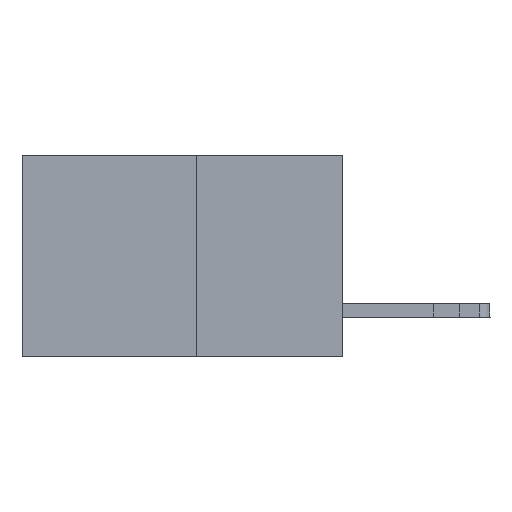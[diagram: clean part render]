
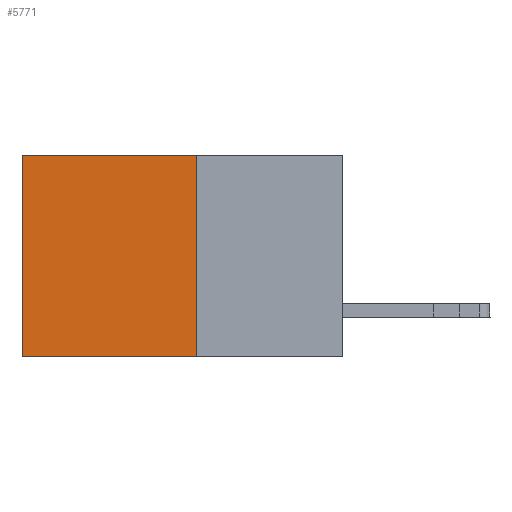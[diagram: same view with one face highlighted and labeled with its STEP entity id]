
A CAD part, left-side view. The second image highlights one B-rep face of the part: STEP entity #5771.
In plain terms, the highlighted planar face has unit normal (-1, 0, 0).
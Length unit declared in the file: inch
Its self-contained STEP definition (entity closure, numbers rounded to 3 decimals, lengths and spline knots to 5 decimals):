
#419 = FACE_OUTER_BOUND ( 'NONE', #8455, .T. ) ;
#1815 = LINE ( 'NONE', #14845, #19613 ) ;
#2249 = VERTEX_POINT ( 'NONE', #11006 ) ;
#2695 = CARTESIAN_POINT ( 'NONE',  ( 0.277, 0.27, -0.37 ) ) ;
#3165 = EDGE_CURVE ( 'NONE', #24280, #2249, #1815, .T. ) ;
#3408 = CARTESIAN_POINT ( 'NONE',  ( 0.277, 0.59, -0.37 ) ) ;
#4039 = EDGE_CURVE ( 'NONE', #24280, #22202, #10521, .T. ) ;
#5771 = ADVANCED_FACE ( 'NONE', ( #419 ), #15603, .F. ) ;
#6904 = LINE ( 'NONE', #11055, #23660 ) ;
#7126 = CARTESIAN_POINT ( 'NONE',  ( 0.277, 0.27, -0.37 ) ) ;
#8455 = EDGE_LOOP ( 'NONE', ( #21153, #15547, #9167, #14128 ) ) ;
#9142 = DIRECTION ( 'NONE',  ( 0., 1., 0. ) ) ;
#9167 = ORIENTED_EDGE ( 'NONE', *, *, #4039, .F. ) ;
#10252 = EDGE_CURVE ( 'NONE', #2249, #18448, #6904, .T. ) ;
#10521 = LINE ( 'NONE', #2695, #21173 ) ;
#11006 = CARTESIAN_POINT ( 'NONE',  ( 0.277, 0.59, 0. ) ) ;
#11055 = CARTESIAN_POINT ( 'NONE',  ( 0.277, 0.59, -0.37 ) ) ;
#11447 = CARTESIAN_POINT ( 'NONE',  ( 0.277, 0.27, -0.37 ) ) ;
#14128 = ORIENTED_EDGE ( 'NONE', *, *, #3165, .T. ) ;
#14845 = CARTESIAN_POINT ( 'NONE',  ( 0.277, 0.27, 0. ) ) ;
#15547 = ORIENTED_EDGE ( 'NONE', *, *, #23198, .F. ) ;
#15603 = PLANE ( 'NONE',  #19559 ) ;
#15862 = DIRECTION ( 'NONE',  ( 1., 0., 0. ) ) ;
#16754 = DIRECTION ( 'NONE',  ( 0., 0., -1. ) ) ;
#17400 = DIRECTION ( 'NONE',  ( 0., 1., 0. ) ) ;
#17988 = DIRECTION ( 'NONE',  ( 0., 0., -1. ) ) ;
#18115 = VECTOR ( 'NONE', #17400, 39.37008 ) ;
#18448 = VERTEX_POINT ( 'NONE', #3408 ) ;
#19559 = AXIS2_PLACEMENT_3D ( 'NONE', #23324, #15862, #23579 ) ;
#19613 = VECTOR ( 'NONE', #9142, 39.37008 ) ;
#21153 = ORIENTED_EDGE ( 'NONE', *, *, #10252, .T. ) ;
#21169 = CARTESIAN_POINT ( 'NONE',  ( 0.277, 0.27, 0. ) ) ;
#21173 = VECTOR ( 'NONE', #17988, 39.37008 ) ;
#22202 = VERTEX_POINT ( 'NONE', #7126 ) ;
#23198 = EDGE_CURVE ( 'NONE', #22202, #18448, #24754, .T. ) ;
#23324 = CARTESIAN_POINT ( 'NONE',  ( 0.277, 0.27, -0.37 ) ) ;
#23579 = DIRECTION ( 'NONE',  ( 0., 0., -1. ) ) ;
#23660 = VECTOR ( 'NONE', #16754, 39.37008 ) ;
#24280 = VERTEX_POINT ( 'NONE', #21169 ) ;
#24754 = LINE ( 'NONE', #11447, #18115 ) ;
